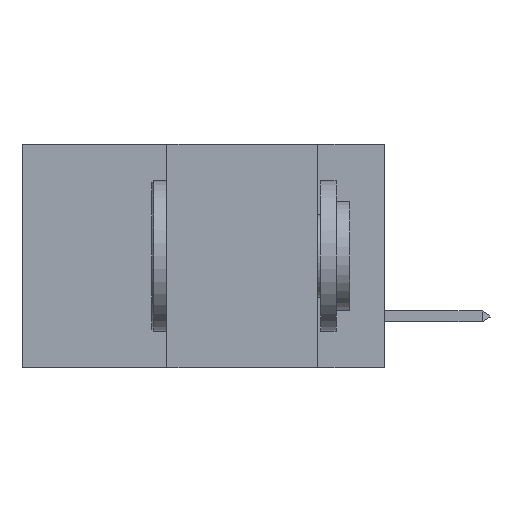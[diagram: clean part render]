
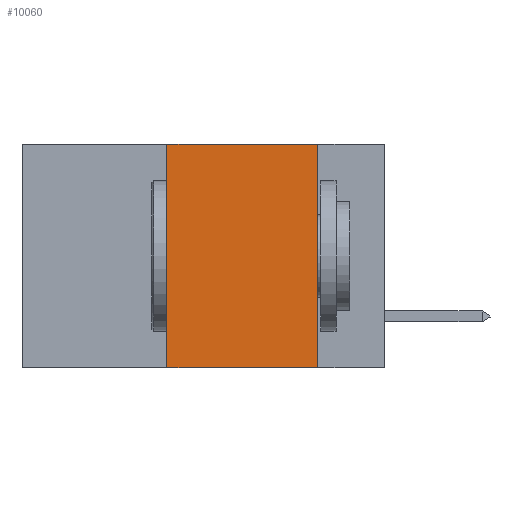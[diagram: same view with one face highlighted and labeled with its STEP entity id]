
A CAD part, left-side view. The second image highlights one B-rep face of the part: STEP entity #10060.
In plain terms, the highlighted planar face has unit normal (-1, 0, 0).
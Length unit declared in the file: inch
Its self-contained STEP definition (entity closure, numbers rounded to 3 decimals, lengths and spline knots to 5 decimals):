
#33 = EDGE_CURVE ( 'NONE', #1931, #8638, #9941, .T. ) ;
#118 = DIRECTION ( 'NONE',  ( 0., 0., -1. ) ) ;
#286 = DIRECTION ( 'NONE',  ( 0., -1., 0. ) ) ;
#360 = VECTOR ( 'NONE', #118, 39.37008 ) ;
#678 = EDGE_LOOP ( 'NONE', ( #7898, #13306, #4783, #4321 ) ) ;
#1412 = EDGE_CURVE ( 'NONE', #5255, #1931, #12242, .T. ) ;
#1721 = VECTOR ( 'NONE', #10321, 39.37008 ) ;
#1841 = CARTESIAN_POINT ( 'NONE',  ( 0., 0.36, 0. ) ) ;
#1931 = VERTEX_POINT ( 'NONE', #9872 ) ;
#2767 = FACE_OUTER_BOUND ( 'NONE', #678, .T. ) ;
#4321 = ORIENTED_EDGE ( 'NONE', *, *, #9237, .T. ) ;
#4783 = ORIENTED_EDGE ( 'NONE', *, *, #14091, .F. ) ;
#5019 = LINE ( 'NONE', #15180, #14998 ) ;
#5255 = VERTEX_POINT ( 'NONE', #1841 ) ;
#6482 = DIRECTION ( 'NONE',  ( 0., -1., 0. ) ) ;
#7343 = AXIS2_PLACEMENT_3D ( 'NONE', #15855, #7732, #13295 ) ;
#7732 = DIRECTION ( 'NONE',  ( 1., 0., 0. ) ) ;
#7898 = ORIENTED_EDGE ( 'NONE', *, *, #33, .F. ) ;
#7962 = VERTEX_POINT ( 'NONE', #11660 ) ;
#8638 = VERTEX_POINT ( 'NONE', #11543 ) ;
#9237 = EDGE_CURVE ( 'NONE', #7962, #8638, #5019, .T. ) ;
#9716 = CARTESIAN_POINT ( 'NONE',  ( 0., 0.11, 0. ) ) ;
#9872 = CARTESIAN_POINT ( 'NONE',  ( 0., 0.11, 0. ) ) ;
#9941 = LINE ( 'NONE', #9716, #360 ) ;
#10060 = ADVANCED_FACE ( 'NONE', ( #2767 ), #14598, .F. ) ;
#10321 = DIRECTION ( 'NONE',  ( 0., 0., 1. ) ) ;
#10349 = CARTESIAN_POINT ( 'NONE',  ( 0., 0.6, 0. ) ) ;
#10430 = CARTESIAN_POINT ( 'NONE',  ( 0., 0.36, 0. ) ) ;
#11543 = CARTESIAN_POINT ( 'NONE',  ( 0., 0.11, -0.37 ) ) ;
#11660 = CARTESIAN_POINT ( 'NONE',  ( 0., 0.36, -0.37 ) ) ;
#12242 = LINE ( 'NONE', #10349, #14576 ) ;
#13295 = DIRECTION ( 'NONE',  ( 0., 0., -1. ) ) ;
#13306 = ORIENTED_EDGE ( 'NONE', *, *, #1412, .F. ) ;
#14091 = EDGE_CURVE ( 'NONE', #7962, #5255, #16204, .T. ) ;
#14576 = VECTOR ( 'NONE', #6482, 39.37008 ) ;
#14598 = PLANE ( 'NONE',  #7343 ) ;
#14998 = VECTOR ( 'NONE', #286, 39.37008 ) ;
#15180 = CARTESIAN_POINT ( 'NONE',  ( 0., 0.6, -0.37 ) ) ;
#15855 = CARTESIAN_POINT ( 'NONE',  ( 0., 0.6, 0. ) ) ;
#16204 = LINE ( 'NONE', #10430, #1721 ) ;
